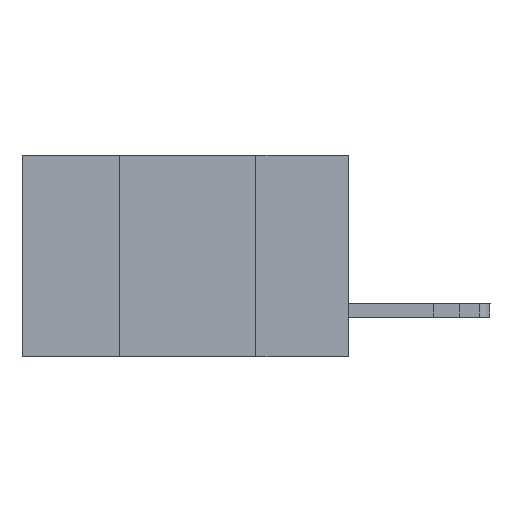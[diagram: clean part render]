
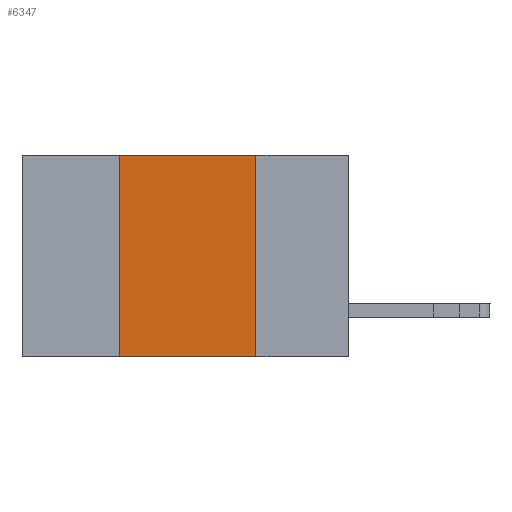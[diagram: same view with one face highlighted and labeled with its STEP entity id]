
A CAD part, left-side view. The second image highlights one B-rep face of the part: STEP entity #6347.
In plain terms, the highlighted planar face has unit normal (-1, 0, 0).
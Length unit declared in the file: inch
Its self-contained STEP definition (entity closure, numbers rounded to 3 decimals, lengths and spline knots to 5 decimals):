
#2640 = EDGE_CURVE ( 'NONE', #10487, #4710, #10933, .T. ) ;
#2866 = VECTOR ( 'NONE', #6993, 39.37008 ) ;
#3191 = LINE ( 'NONE', #10985, #12285 ) ;
#3227 = LINE ( 'NONE', #7044, #2866 ) ;
#3435 = EDGE_CURVE ( 'NONE', #12096, #10487, #3227, .T. ) ;
#3916 = EDGE_CURVE ( 'NONE', #10259, #4710, #6239, .T. ) ;
#4710 = VERTEX_POINT ( 'NONE', #15023 ) ;
#5136 = DIRECTION ( 'NONE',  ( 0., -1., 0. ) ) ;
#5454 = CARTESIAN_POINT ( 'NONE',  ( 0., 0.6, -0.37 ) ) ;
#5518 = EDGE_CURVE ( 'NONE', #10259, #12096, #3191, .T. ) ;
#6239 = LINE ( 'NONE', #5454, #9138 ) ;
#6347 = ADVANCED_FACE ( 'NONE', ( #11565 ), #14064, .F. ) ;
#6993 = DIRECTION ( 'NONE',  ( 0., -1., 0. ) ) ;
#7044 = CARTESIAN_POINT ( 'NONE',  ( 0., 0.6, 0. ) ) ;
#7299 = CARTESIAN_POINT ( 'NONE',  ( 0., 0.42, -0.37 ) ) ;
#7579 = ORIENTED_EDGE ( 'NONE', *, *, #5518, .F. ) ;
#8936 = CARTESIAN_POINT ( 'NONE',  ( 0., 0.17, 0. ) ) ;
#9138 = VECTOR ( 'NONE', #5136, 39.37008 ) ;
#10009 = AXIS2_PLACEMENT_3D ( 'NONE', #14449, #14069, #14085 ) ;
#10259 = VERTEX_POINT ( 'NONE', #7299 ) ;
#10487 = VERTEX_POINT ( 'NONE', #8936 ) ;
#10714 = ORIENTED_EDGE ( 'NONE', *, *, #3435, .F. ) ;
#10933 = LINE ( 'NONE', #14391, #13570 ) ;
#10985 = CARTESIAN_POINT ( 'NONE',  ( 0., 0.42, -0.37 ) ) ;
#11065 = ORIENTED_EDGE ( 'NONE', *, *, #2640, .F. ) ;
#11070 = DIRECTION ( 'NONE',  ( 0., 0., 1. ) ) ;
#11484 = CARTESIAN_POINT ( 'NONE',  ( 0., 0.42, 0. ) ) ;
#11565 = FACE_OUTER_BOUND ( 'NONE', #14914, .T. ) ;
#12096 = VERTEX_POINT ( 'NONE', #11484 ) ;
#12285 = VECTOR ( 'NONE', #11070, 39.37008 ) ;
#13356 = ORIENTED_EDGE ( 'NONE', *, *, #3916, .T. ) ;
#13550 = DIRECTION ( 'NONE',  ( 0., 0., -1. ) ) ;
#13570 = VECTOR ( 'NONE', #13550, 39.37008 ) ;
#14064 = PLANE ( 'NONE',  #10009 ) ;
#14069 = DIRECTION ( 'NONE',  ( 1., 0., 0. ) ) ;
#14085 = DIRECTION ( 'NONE',  ( 0., 0., -1. ) ) ;
#14391 = CARTESIAN_POINT ( 'NONE',  ( 0., 0.17, -0.37 ) ) ;
#14449 = CARTESIAN_POINT ( 'NONE',  ( 0., 0.6, 0. ) ) ;
#14914 = EDGE_LOOP ( 'NONE', ( #11065, #10714, #7579, #13356 ) ) ;
#15023 = CARTESIAN_POINT ( 'NONE',  ( 0., 0.17, -0.37 ) ) ;
